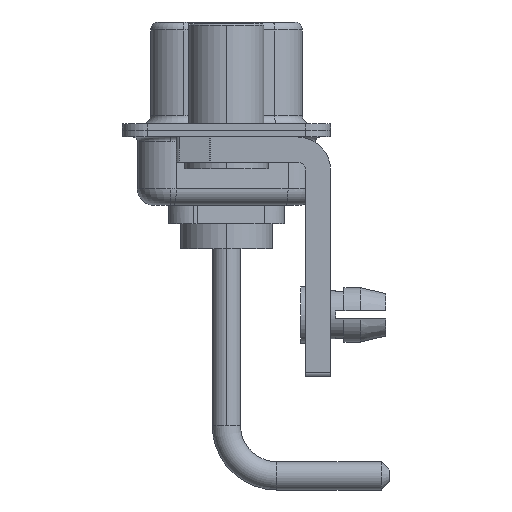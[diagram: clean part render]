
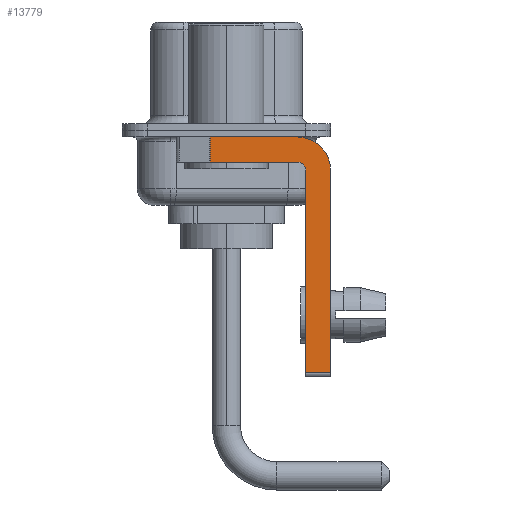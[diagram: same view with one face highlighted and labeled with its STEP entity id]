
A CAD part, left-side view. The second image highlights one B-rep face of the part: STEP entity #13779.
In plain terms, the highlighted planar face has unit normal (-1, 0, 0).
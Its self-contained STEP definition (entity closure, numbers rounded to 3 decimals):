
#19 = DIRECTION ( 'NONE',  ( -1., 0., 0. ) ) ;
#559 = ORIENTED_EDGE ( 'NONE', *, *, #8163, .T. ) ;
#797 = VECTOR ( 'NONE', #10754, 1000. ) ;
#970 = ORIENTED_EDGE ( 'NONE', *, *, #15287, .F. ) ;
#1214 = ORIENTED_EDGE ( 'NONE', *, *, #9530, .F. ) ;
#2351 = VECTOR ( 'NONE', #15788, 1000. ) ;
#2785 = EDGE_CURVE ( 'NONE', #4868, #8818, #3292, .T. ) ;
#3142 = DIRECTION ( 'NONE',  ( 0., 0., 1. ) ) ;
#3292 = LINE ( 'NONE', #20037, #2351 ) ;
#3544 = CARTESIAN_POINT ( 'NONE',  ( -2.9, -4.25, -14.55 ) ) ;
#3832 = ORIENTED_EDGE ( 'NONE', *, *, #2785, .F. ) ;
#4003 = ORIENTED_EDGE ( 'NONE', *, *, #14279, .T. ) ;
#4154 = VECTOR ( 'NONE', #7901, 1000. ) ;
#4868 = VERTEX_POINT ( 'NONE', #7508 ) ;
#5084 = DIRECTION ( 'NONE',  ( 0., 0., -1. ) ) ;
#5418 = ORIENTED_EDGE ( 'NONE', *, *, #7635, .F. ) ;
#6330 = CARTESIAN_POINT ( 'NONE',  ( -2.9, -4.25, -2.4 ) ) ;
#7344 = VECTOR ( 'NONE', #7922, 1000. ) ;
#7508 = CARTESIAN_POINT ( 'NONE',  ( -2.9, -6.25, -2.4 ) ) ;
#7635 = EDGE_CURVE ( 'NONE', #19382, #7752, #18640, .T. ) ;
#7647 = ORIENTED_EDGE ( 'NONE', *, *, #9662, .F. ) ;
#7752 = VERTEX_POINT ( 'NONE', #8183 ) ;
#7901 = DIRECTION ( 'NONE',  ( 0., 0., -1. ) ) ;
#7922 = DIRECTION ( 'NONE',  ( 0., -1., 0. ) ) ;
#8163 = EDGE_CURVE ( 'NONE', #10182, #8818, #17573, .T. ) ;
#8183 = CARTESIAN_POINT ( 'NONE',  ( -2.9, 0.978, -1.9 ) ) ;
#8334 = FACE_OUTER_BOUND ( 'NONE', #11118, .T. ) ;
#8786 = VERTEX_POINT ( 'NONE', #17929 ) ;
#8818 = VERTEX_POINT ( 'NONE', #14963 ) ;
#9097 = CARTESIAN_POINT ( 'NONE',  ( -2.9, -4.75, -14.55 ) ) ;
#9342 = CARTESIAN_POINT ( 'NONE',  ( -2.9, 3., -0.4 ) ) ;
#9530 = EDGE_CURVE ( 'NONE', #15074, #4868, #18745, .T. ) ;
#9622 = CARTESIAN_POINT ( 'NONE',  ( -2.9, 0.978, -1.9 ) ) ;
#9662 = EDGE_CURVE ( 'NONE', #10182, #14620, #13147, .T. ) ;
#10182 = VERTEX_POINT ( 'NONE', #9097 ) ;
#10298 = CARTESIAN_POINT ( 'NONE',  ( -2.9, -4.25, -0.4 ) ) ;
#10754 = DIRECTION ( 'NONE',  ( 0., 0., 1. ) ) ;
#10944 = AXIS2_PLACEMENT_3D ( 'NONE', #14285, #11290, #5084 ) ;
#10988 = AXIS2_PLACEMENT_3D ( 'NONE', #6330, #19, #3142 ) ;
#11118 = EDGE_LOOP ( 'NONE', ( #17445, #4003, #5418, #970, #7647, #559, #3832, #1214 ) ) ;
#11290 = DIRECTION ( 'NONE',  ( 1., 0., 0. ) ) ;
#12157 = DIRECTION ( 'NONE',  ( 0., 0., -1. ) ) ;
#12233 = VECTOR ( 'NONE', #15572, 1000. ) ;
#12453 = CARTESIAN_POINT ( 'NONE',  ( -2.9, -4.25, -2.4 ) ) ;
#12582 = EDGE_CURVE ( 'NONE', #8786, #15074, #17156, .T. ) ;
#13147 = LINE ( 'NONE', #15199, #797 ) ;
#13523 = CARTESIAN_POINT ( 'NONE',  ( -2.9, -4.75, -2.4 ) ) ;
#13635 = CIRCLE ( 'NONE', #10988, 0.5 ) ;
#13779 = ADVANCED_FACE ( 'NONE', ( #8334 ), #19109, .F. ) ;
#14279 = EDGE_CURVE ( 'NONE', #8786, #7752, #15793, .T. ) ;
#14285 = CARTESIAN_POINT ( 'NONE',  ( -2.9, -4.25, -2.4 ) ) ;
#14620 = VERTEX_POINT ( 'NONE', #13523 ) ;
#14963 = CARTESIAN_POINT ( 'NONE',  ( -2.9, -6.25, -14.55 ) ) ;
#15074 = VERTEX_POINT ( 'NONE', #10298 ) ;
#15199 = CARTESIAN_POINT ( 'NONE',  ( -2.9, -4.75, -14.8 ) ) ;
#15287 = EDGE_CURVE ( 'NONE', #14620, #19382, #13635, .T. ) ;
#15572 = DIRECTION ( 'NONE',  ( 0., 1., 0. ) ) ;
#15640 = DIRECTION ( 'NONE',  ( 0., -1., 0. ) ) ;
#15782 = VECTOR ( 'NONE', #15640, 1000. ) ;
#15788 = DIRECTION ( 'NONE',  ( 0., 0., -1. ) ) ;
#15793 = LINE ( 'NONE', #9622, #4154 ) ;
#16792 = DIRECTION ( 'NONE',  ( 1., 0., 0. ) ) ;
#17156 = LINE ( 'NONE', #9342, #7344 ) ;
#17445 = ORIENTED_EDGE ( 'NONE', *, *, #12582, .F. ) ;
#17573 = LINE ( 'NONE', #3544, #15782 ) ;
#17929 = CARTESIAN_POINT ( 'NONE',  ( -2.9, 0.978, -0.4 ) ) ;
#18640 = LINE ( 'NONE', #18742, #12233 ) ;
#18742 = CARTESIAN_POINT ( 'NONE',  ( -2.9, -4.25, -1.9 ) ) ;
#18745 = CIRCLE ( 'NONE', #20094, 2. ) ;
#19109 = PLANE ( 'NONE',  #10944 ) ;
#19382 = VERTEX_POINT ( 'NONE', #19891 ) ;
#19891 = CARTESIAN_POINT ( 'NONE',  ( -2.9, -4.25, -1.9 ) ) ;
#20037 = CARTESIAN_POINT ( 'NONE',  ( -2.9, -6.25, -2.4 ) ) ;
#20094 = AXIS2_PLACEMENT_3D ( 'NONE', #12453, #16792, #12157 ) ;
